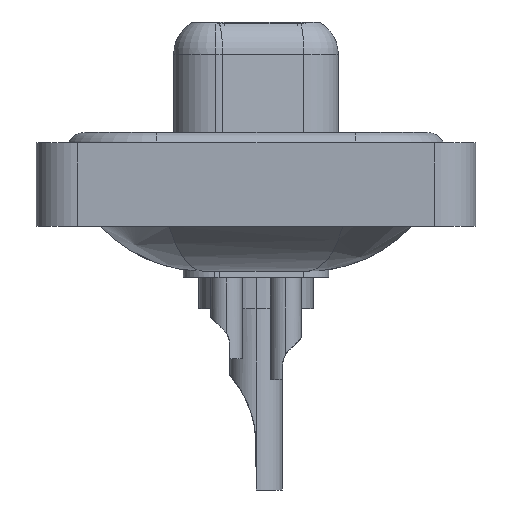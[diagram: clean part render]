
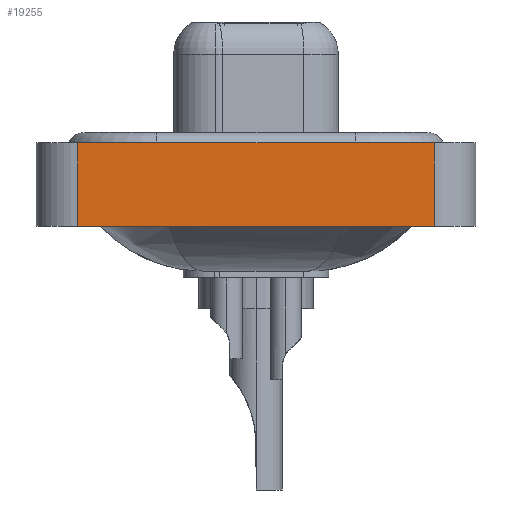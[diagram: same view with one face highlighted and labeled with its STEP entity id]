
A CAD part, left-side view. The second image highlights one B-rep face of the part: STEP entity #19255.
In plain terms, the highlighted planar face has unit normal (-1, 0, 0).
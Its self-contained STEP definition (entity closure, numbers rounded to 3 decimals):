
#711 = EDGE_CURVE ( 'NONE', #18946, #22119, #16802, .T. ) ;
#2454 = CARTESIAN_POINT ( 'NONE',  ( -7.3, -8.55, -3.6 ) ) ;
#2769 = FACE_OUTER_BOUND ( 'NONE', #22373, .T. ) ;
#2867 = DIRECTION ( 'NONE',  ( 0., -1., 0. ) ) ;
#3029 = VECTOR ( 'NONE', #19347, 1000. ) ;
#5066 = DIRECTION ( 'NONE',  ( 0., 0., 1. ) ) ;
#6279 = DIRECTION ( 'NONE',  ( -1., 0., 0. ) ) ;
#6563 = VECTOR ( 'NONE', #9879, 1000. ) ;
#7427 = CARTESIAN_POINT ( 'NONE',  ( -7.3, 8.55, 0.4 ) ) ;
#7465 = ORIENTED_EDGE ( 'NONE', *, *, #22015, .T. ) ;
#7903 = ORIENTED_EDGE ( 'NONE', *, *, #17237, .F. ) ;
#9257 = DIRECTION ( 'NONE',  ( 0., 0., 1. ) ) ;
#9367 = PLANE ( 'NONE',  #17569 ) ;
#9545 = LINE ( 'NONE', #21972, #6563 ) ;
#9879 = DIRECTION ( 'NONE',  ( 0., 0., 1. ) ) ;
#10309 = LINE ( 'NONE', #22283, #11860 ) ;
#11201 = ORIENTED_EDGE ( 'NONE', *, *, #20423, .T. ) ;
#11860 = VECTOR ( 'NONE', #5066, 1000. ) ;
#13525 = CARTESIAN_POINT ( 'NONE',  ( -7.3, -8.55, 0.4 ) ) ;
#13641 = CARTESIAN_POINT ( 'NONE',  ( -7.3, 8.55, -3.6 ) ) ;
#16802 = LINE ( 'NONE', #13525, #17652 ) ;
#16914 = VERTEX_POINT ( 'NONE', #13641 ) ;
#17237 = EDGE_CURVE ( 'NONE', #16914, #18946, #9545, .T. ) ;
#17374 = ORIENTED_EDGE ( 'NONE', *, *, #711, .F. ) ;
#17569 = AXIS2_PLACEMENT_3D ( 'NONE', #21778, #6279, #9257 ) ;
#17652 = VECTOR ( 'NONE', #2867, 1000. ) ;
#17983 = LINE ( 'NONE', #2454, #3029 ) ;
#18706 = CARTESIAN_POINT ( 'NONE',  ( -7.3, -8.55, -3.6 ) ) ;
#18946 = VERTEX_POINT ( 'NONE', #7427 ) ;
#19255 = ADVANCED_FACE ( 'NONE', ( #2769 ), #9367, .T. ) ;
#19347 = DIRECTION ( 'NONE',  ( 0., -1., 0. ) ) ;
#19643 = VERTEX_POINT ( 'NONE', #18706 ) ;
#20423 = EDGE_CURVE ( 'NONE', #19643, #22119, #10309, .T. ) ;
#21778 = CARTESIAN_POINT ( 'NONE',  ( -7.3, -8.55, -3.6 ) ) ;
#21972 = CARTESIAN_POINT ( 'NONE',  ( -7.3, 8.55, -3.6 ) ) ;
#22015 = EDGE_CURVE ( 'NONE', #16914, #19643, #17983, .T. ) ;
#22119 = VERTEX_POINT ( 'NONE', #22367 ) ;
#22283 = CARTESIAN_POINT ( 'NONE',  ( -7.3, -8.55, -3.6 ) ) ;
#22367 = CARTESIAN_POINT ( 'NONE',  ( -7.3, -8.55, 0.4 ) ) ;
#22373 = EDGE_LOOP ( 'NONE', ( #11201, #17374, #7903, #7465 ) ) ;
